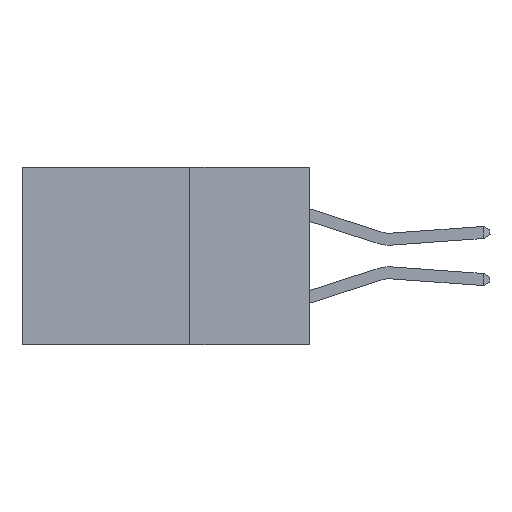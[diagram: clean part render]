
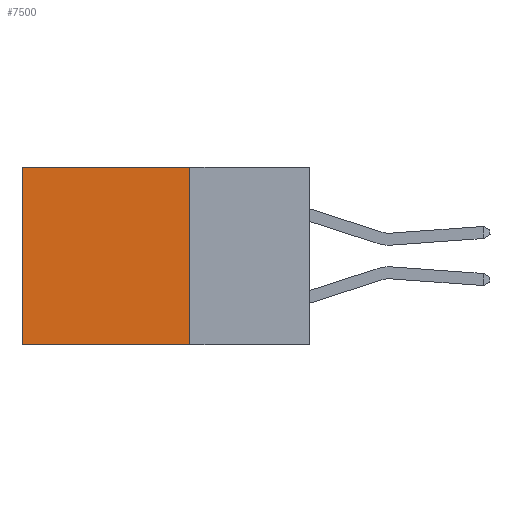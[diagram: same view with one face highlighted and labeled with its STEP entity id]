
A CAD part, left-side view. The second image highlights one B-rep face of the part: STEP entity #7500.
In plain terms, the highlighted planar face has unit normal (-1, 0, 0).
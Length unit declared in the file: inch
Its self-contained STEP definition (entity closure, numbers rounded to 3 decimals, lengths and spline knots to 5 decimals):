
#557 = CARTESIAN_POINT ( 'NONE',  ( 0.2615, 0.25, -0.37 ) ) ;
#719 = CARTESIAN_POINT ( 'NONE',  ( 0.2615, 0.25, -0.37 ) ) ;
#845 = FACE_OUTER_BOUND ( 'NONE', #1971, .T. ) ;
#1949 = ORIENTED_EDGE ( 'NONE', *, *, #12724, .T. ) ;
#1971 = EDGE_LOOP ( 'NONE', ( #5086, #13607, #15406, #1949 ) ) ;
#2279 = CARTESIAN_POINT ( 'NONE',  ( 0.2615, 0.25, 0. ) ) ;
#3622 = DIRECTION ( 'NONE',  ( 0., 1., 0. ) ) ;
#3659 = EDGE_CURVE ( 'NONE', #15950, #11457, #14571, .T. ) ;
#4698 = VECTOR ( 'NONE', #6330, 39.37008 ) ;
#5086 = ORIENTED_EDGE ( 'NONE', *, *, #16293, .T. ) ;
#5397 = VECTOR ( 'NONE', #6502, 39.37008 ) ;
#6330 = DIRECTION ( 'NONE',  ( 0., 0., -1. ) ) ;
#6360 = DIRECTION ( 'NONE',  ( 0., 0., -1. ) ) ;
#6502 = DIRECTION ( 'NONE',  ( 0., 1., 0. ) ) ;
#6551 = VERTEX_POINT ( 'NONE', #17537 ) ;
#6708 = CARTESIAN_POINT ( 'NONE',  ( 0.2615, 0.6, 0. ) ) ;
#7500 = ADVANCED_FACE ( 'NONE', ( #845 ), #9181, .F. ) ;
#7912 = DIRECTION ( 'NONE',  ( 1., 0., 0. ) ) ;
#8277 = AXIS2_PLACEMENT_3D ( 'NONE', #15964, #7912, #6360 ) ;
#8439 = EDGE_CURVE ( 'NONE', #6551, #15950, #11765, .T. ) ;
#9181 = PLANE ( 'NONE',  #8277 ) ;
#10327 = CARTESIAN_POINT ( 'NONE',  ( 0.2615, 0.25, -0.37 ) ) ;
#10386 = VECTOR ( 'NONE', #15783, 39.37008 ) ;
#10459 = LINE ( 'NONE', #13351, #10386 ) ;
#10715 = VERTEX_POINT ( 'NONE', #6708 ) ;
#11331 = VECTOR ( 'NONE', #3622, 39.37008 ) ;
#11457 = VERTEX_POINT ( 'NONE', #16096 ) ;
#11765 = LINE ( 'NONE', #10327, #4698 ) ;
#12724 = EDGE_CURVE ( 'NONE', #6551, #10715, #14491, .T. ) ;
#13351 = CARTESIAN_POINT ( 'NONE',  ( 0.2615, 0.6, -0.37 ) ) ;
#13607 = ORIENTED_EDGE ( 'NONE', *, *, #3659, .F. ) ;
#14491 = LINE ( 'NONE', #2279, #11331 ) ;
#14571 = LINE ( 'NONE', #719, #5397 ) ;
#15406 = ORIENTED_EDGE ( 'NONE', *, *, #8439, .F. ) ;
#15783 = DIRECTION ( 'NONE',  ( 0., 0., -1. ) ) ;
#15950 = VERTEX_POINT ( 'NONE', #557 ) ;
#15964 = CARTESIAN_POINT ( 'NONE',  ( 0.2615, 0.25, -0.37 ) ) ;
#16096 = CARTESIAN_POINT ( 'NONE',  ( 0.2615, 0.6, -0.37 ) ) ;
#16293 = EDGE_CURVE ( 'NONE', #10715, #11457, #10459, .T. ) ;
#17537 = CARTESIAN_POINT ( 'NONE',  ( 0.2615, 0.25, 0. ) ) ;
